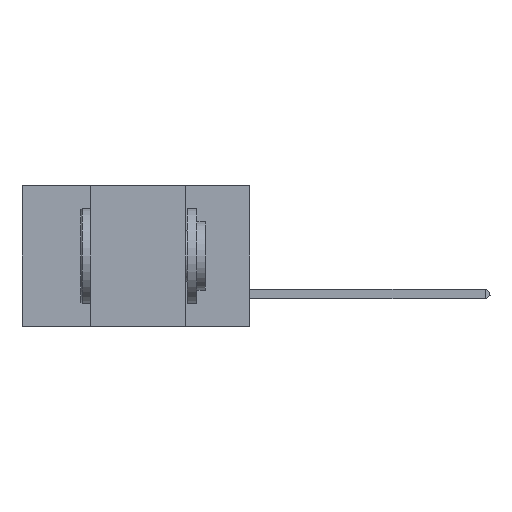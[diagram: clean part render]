
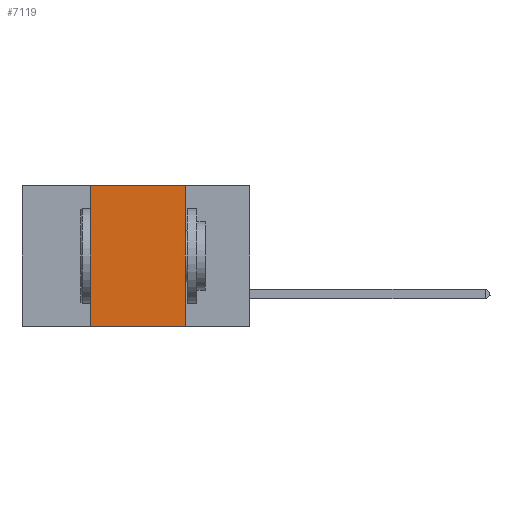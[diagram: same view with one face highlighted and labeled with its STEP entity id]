
A CAD part, left-side view. The second image highlights one B-rep face of the part: STEP entity #7119.
In plain terms, the highlighted planar face has unit normal (-1, 0, 0).
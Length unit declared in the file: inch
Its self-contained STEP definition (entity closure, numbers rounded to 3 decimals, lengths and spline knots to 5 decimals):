
#326 = EDGE_LOOP ( 'NONE', ( #23741, #43547, #11172, #21695 ) ) ;
#1824 = DIRECTION ( 'NONE',  ( 0., 0., -1. ) ) ;
#1866 = CARTESIAN_POINT ( 'NONE',  ( 0., 0.42, 0. ) ) ;
#2075 = CARTESIAN_POINT ( 'NONE',  ( 0., 0.17, 0. ) ) ;
#4905 = EDGE_CURVE ( 'NONE', #26532, #23329, #32695, .T. ) ;
#6875 = CARTESIAN_POINT ( 'NONE',  ( 0., 0.17, 0. ) ) ;
#7119 = ADVANCED_FACE ( 'NONE', ( #17690 ), #40194, .F. ) ;
#8302 = LINE ( 'NONE', #31662, #38557 ) ;
#10404 = DIRECTION ( 'NONE',  ( 0., 0., 1. ) ) ;
#10941 = CARTESIAN_POINT ( 'NONE',  ( 0., 0.42, -0.37 ) ) ;
#11172 = ORIENTED_EDGE ( 'NONE', *, *, #43695, .F. ) ;
#11778 = VECTOR ( 'NONE', #30240, 39.37008 ) ;
#11944 = CARTESIAN_POINT ( 'NONE',  ( 0., 0.42, 0. ) ) ;
#17621 = AXIS2_PLACEMENT_3D ( 'NONE', #43684, #22853, #1824 ) ;
#17690 = FACE_OUTER_BOUND ( 'NONE', #326, .T. ) ;
#21383 = EDGE_CURVE ( 'NONE', #40103, #24564, #8302, .T. ) ;
#21695 = ORIENTED_EDGE ( 'NONE', *, *, #4905, .T. ) ;
#22853 = DIRECTION ( 'NONE',  ( 1., 0., 0. ) ) ;
#23329 = VERTEX_POINT ( 'NONE', #35268 ) ;
#23741 = ORIENTED_EDGE ( 'NONE', *, *, #25841, .F. ) ;
#23784 = DIRECTION ( 'NONE',  ( 0., 0., -1. ) ) ;
#24564 = VERTEX_POINT ( 'NONE', #2075 ) ;
#24908 = LINE ( 'NONE', #6875, #45294 ) ;
#25060 = DIRECTION ( 'NONE',  ( 0., -1., 0. ) ) ;
#25841 = EDGE_CURVE ( 'NONE', #24564, #23329, #24908, .T. ) ;
#26532 = VERTEX_POINT ( 'NONE', #10941 ) ;
#30240 = DIRECTION ( 'NONE',  ( 0., -1., 0. ) ) ;
#31662 = CARTESIAN_POINT ( 'NONE',  ( 0., 0.6, 0. ) ) ;
#32695 = LINE ( 'NONE', #45364, #11778 ) ;
#35019 = VECTOR ( 'NONE', #10404, 39.37008 ) ;
#35268 = CARTESIAN_POINT ( 'NONE',  ( 0., 0.17, -0.37 ) ) ;
#38557 = VECTOR ( 'NONE', #25060, 39.37008 ) ;
#39887 = LINE ( 'NONE', #11944, #35019 ) ;
#40103 = VERTEX_POINT ( 'NONE', #1866 ) ;
#40194 = PLANE ( 'NONE',  #17621 ) ;
#43547 = ORIENTED_EDGE ( 'NONE', *, *, #21383, .F. ) ;
#43684 = CARTESIAN_POINT ( 'NONE',  ( 0., 0.6, 0. ) ) ;
#43695 = EDGE_CURVE ( 'NONE', #26532, #40103, #39887, .T. ) ;
#45294 = VECTOR ( 'NONE', #23784, 39.37008 ) ;
#45364 = CARTESIAN_POINT ( 'NONE',  ( 0., 0.6, -0.37 ) ) ;
